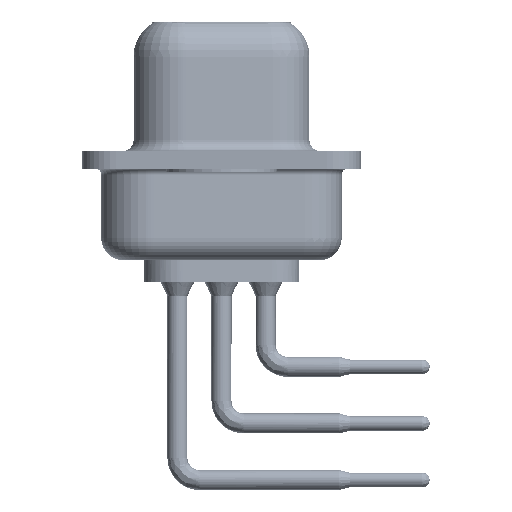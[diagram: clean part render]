
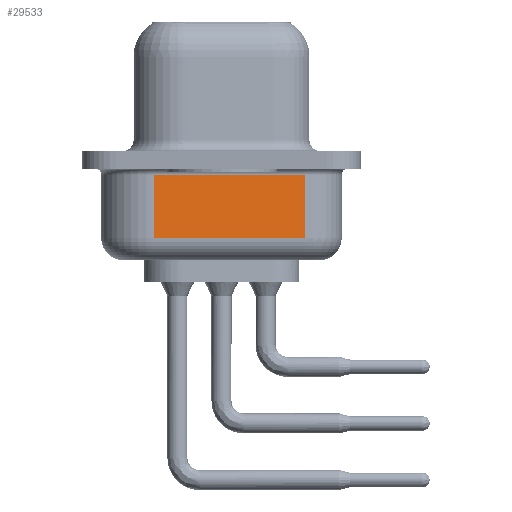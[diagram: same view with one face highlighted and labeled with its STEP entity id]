
A CAD part, left-side view. The second image highlights one B-rep face of the part: STEP entity #29533.
In plain terms, the highlighted planar face has unit normal (-0.985, -0.174, 0).
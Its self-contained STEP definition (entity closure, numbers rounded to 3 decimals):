
#1612 = LINE ( 'NONE', #22565, #8234 ) ;
#3659 = VECTOR ( 'NONE', #4656, 1000. ) ;
#3694 = VERTEX_POINT ( 'NONE', #26366 ) ;
#4526 = LINE ( 'NONE', #28905, #19421 ) ;
#4582 = LINE ( 'NONE', #21411, #3659 ) ;
#4656 = DIRECTION ( 'NONE',  ( 0.174, -0.985, 0. ) ) ;
#7580 = CARTESIAN_POINT ( 'NONE',  ( 2.88, 3.053, -3.5 ) ) ;
#7784 = CARTESIAN_POINT ( 'NONE',  ( 4.079, -3.747, -3.5 ) ) ;
#8234 = VECTOR ( 'NONE', #19921, 1000. ) ;
#11633 = AXIS2_PLACEMENT_3D ( 'NONE', #20710, #15230, #34646 ) ;
#13196 = LINE ( 'NONE', #28994, #19749 ) ;
#14022 = EDGE_LOOP ( 'NONE', ( #23558, #34988, #16353, #31538 ) ) ;
#15230 = DIRECTION ( 'NONE',  ( 0.985, 0.174, 0. ) ) ;
#16353 = ORIENTED_EDGE ( 'NONE', *, *, #23115, .T. ) ;
#19410 = EDGE_CURVE ( 'NONE', #3694, #29297, #4526, .T. ) ;
#19421 = VECTOR ( 'NONE', #31679, 1000. ) ;
#19749 = VECTOR ( 'NONE', #31770, 1000. ) ;
#19921 = DIRECTION ( 'NONE',  ( 0., 0., 1. ) ) ;
#20710 = CARTESIAN_POINT ( 'NONE',  ( 2.88, 3.053, -4.5 ) ) ;
#21411 = CARTESIAN_POINT ( 'NONE',  ( 2.88, 3.053, -3.5 ) ) ;
#21494 = EDGE_CURVE ( 'NONE', #32116, #29297, #13196, .T. ) ;
#22565 = CARTESIAN_POINT ( 'NONE',  ( 4.079, -3.747, -4.5 ) ) ;
#23115 = EDGE_CURVE ( 'NONE', #23515, #3694, #1612, .T. ) ;
#23515 = VERTEX_POINT ( 'NONE', #7784 ) ;
#23558 = ORIENTED_EDGE ( 'NONE', *, *, #21494, .F. ) ;
#26166 = EDGE_CURVE ( 'NONE', #32116, #23515, #4582, .T. ) ;
#26289 = PLANE ( 'NONE',  #11633 ) ;
#26366 = CARTESIAN_POINT ( 'NONE',  ( 4.079, -3.747, -0.65 ) ) ;
#28905 = CARTESIAN_POINT ( 'NONE',  ( 2.88, 3.053, -0.65 ) ) ;
#28994 = CARTESIAN_POINT ( 'NONE',  ( 2.88, 3.053, -4.5 ) ) ;
#29297 = VERTEX_POINT ( 'NONE', #34328 ) ;
#29533 = ADVANCED_FACE ( 'NONE', ( #31777 ), #26289, .F. ) ;
#31538 = ORIENTED_EDGE ( 'NONE', *, *, #19410, .T. ) ;
#31679 = DIRECTION ( 'NONE',  ( -0.174, 0.985, 0. ) ) ;
#31770 = DIRECTION ( 'NONE',  ( 0., 0., 1. ) ) ;
#31777 = FACE_OUTER_BOUND ( 'NONE', #14022, .T. ) ;
#32116 = VERTEX_POINT ( 'NONE', #7580 ) ;
#34328 = CARTESIAN_POINT ( 'NONE',  ( 2.88, 3.053, -0.65 ) ) ;
#34646 = DIRECTION ( 'NONE',  ( -0.174, 0.985, 0. ) ) ;
#34988 = ORIENTED_EDGE ( 'NONE', *, *, #26166, .T. ) ;
